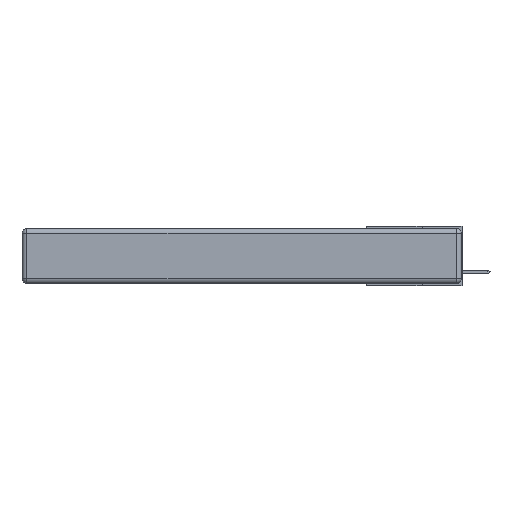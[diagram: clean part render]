
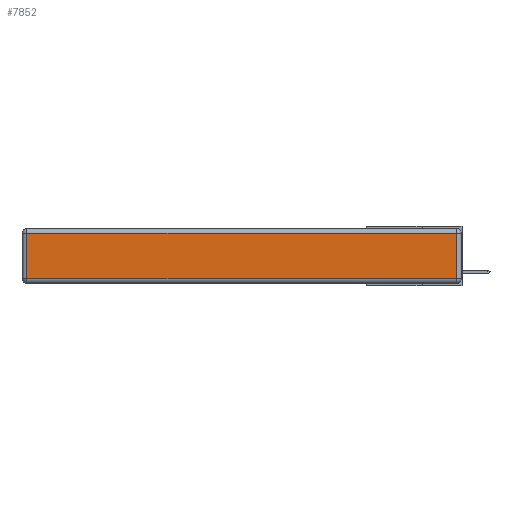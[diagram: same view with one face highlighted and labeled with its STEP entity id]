
A CAD part, left-side view. The second image highlights one B-rep face of the part: STEP entity #7852.
In plain terms, the highlighted planar face has unit normal (-1, 0, 0).
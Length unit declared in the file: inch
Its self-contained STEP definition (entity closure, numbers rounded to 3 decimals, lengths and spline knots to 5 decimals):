
#1 = EDGE_CURVE ( 'NONE', #9278, #3682, #6369, .T. ) ;
#131 = DIRECTION ( 'NONE',  ( 0., 0., -1. ) ) ;
#231 = VERTEX_POINT ( 'NONE', #12543 ) ;
#543 = EDGE_CURVE ( 'NONE', #3682, #3294, #5556, .T. ) ;
#1301 = ORIENTED_EDGE ( 'NONE', *, *, #543, .T. ) ;
#1643 = CARTESIAN_POINT ( 'NONE',  ( 0., 0.03, -0.313 ) ) ;
#2579 = CARTESIAN_POINT ( 'NONE',  ( 0., 2.72, -0.03 ) ) ;
#2764 = DIRECTION ( 'NONE',  ( 0., 1., 0. ) ) ;
#3294 = VERTEX_POINT ( 'NONE', #1643 ) ;
#3366 = VECTOR ( 'NONE', #2764, 39.37008 ) ;
#3531 = FACE_OUTER_BOUND ( 'NONE', #9204, .T. ) ;
#3682 = VERTEX_POINT ( 'NONE', #8046 ) ;
#3731 = CARTESIAN_POINT ( 'NONE',  ( 0., 2.75, -0.03 ) ) ;
#4290 = VECTOR ( 'NONE', #5761, 39.37008 ) ;
#4842 = ORIENTED_EDGE ( 'NONE', *, *, #7837, .T. ) ;
#5439 = EDGE_CURVE ( 'NONE', #3294, #231, #13188, .T. ) ;
#5556 = LINE ( 'NONE', #11551, #8408 ) ;
#5565 = VECTOR ( 'NONE', #131, 39.37008 ) ;
#5761 = DIRECTION ( 'NONE',  ( 0., 0., 1. ) ) ;
#6369 = LINE ( 'NONE', #11138, #5565 ) ;
#6492 = CARTESIAN_POINT ( 'NONE',  ( 0., 0.03, -0.343 ) ) ;
#6679 = DIRECTION ( 'NONE',  ( -1., 0., 0. ) ) ;
#7356 = LINE ( 'NONE', #3731, #3366 ) ;
#7709 = CARTESIAN_POINT ( 'NONE',  ( 0., 0., -0.343 ) ) ;
#7837 = EDGE_CURVE ( 'NONE', #231, #9278, #7356, .T. ) ;
#7838 = PLANE ( 'NONE',  #12183 ) ;
#7852 = ADVANCED_FACE ( 'NONE', ( #3531 ), #7838, .T. ) ;
#8046 = CARTESIAN_POINT ( 'NONE',  ( 0., 2.72, -0.313 ) ) ;
#8408 = VECTOR ( 'NONE', #9491, 39.37008 ) ;
#9204 = EDGE_LOOP ( 'NONE', ( #1301, #11215, #4842, #9218 ) ) ;
#9218 = ORIENTED_EDGE ( 'NONE', *, *, #1, .T. ) ;
#9278 = VERTEX_POINT ( 'NONE', #2579 ) ;
#9491 = DIRECTION ( 'NONE',  ( 0., -1., 0. ) ) ;
#11138 = CARTESIAN_POINT ( 'NONE',  ( 0., 2.72, -0.343 ) ) ;
#11215 = ORIENTED_EDGE ( 'NONE', *, *, #5439, .T. ) ;
#11551 = CARTESIAN_POINT ( 'NONE',  ( 0., 0., -0.313 ) ) ;
#12183 = AXIS2_PLACEMENT_3D ( 'NONE', #7709, #6679, #12810 ) ;
#12543 = CARTESIAN_POINT ( 'NONE',  ( 0., 0.03, -0.03 ) ) ;
#12810 = DIRECTION ( 'NONE',  ( 0., 0., 1. ) ) ;
#13188 = LINE ( 'NONE', #6492, #4290 ) ;
